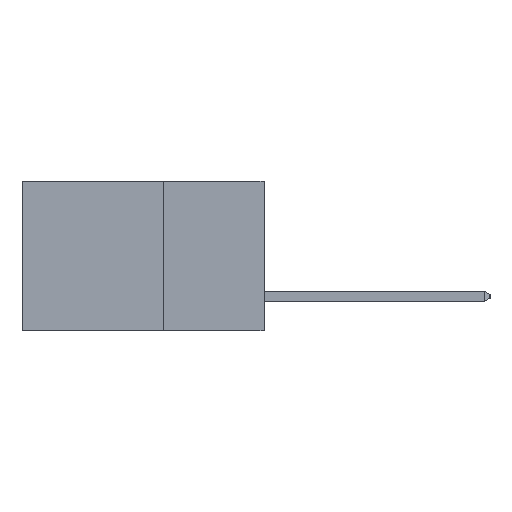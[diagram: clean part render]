
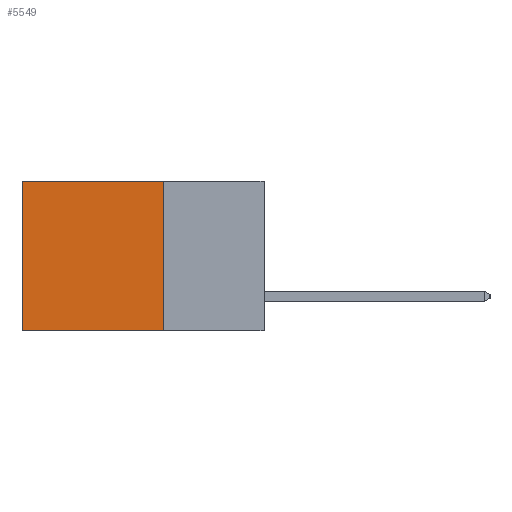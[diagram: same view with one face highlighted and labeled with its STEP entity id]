
A CAD part, left-side view. The second image highlights one B-rep face of the part: STEP entity #5549.
In plain terms, the highlighted planar face has unit normal (-1, 0, 0).
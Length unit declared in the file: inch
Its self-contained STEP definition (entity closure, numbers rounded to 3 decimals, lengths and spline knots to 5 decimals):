
#2765 = CARTESIAN_POINT ( 'NONE',  ( 0.298, 0.6, 0. ) ) ;
#3063 = CARTESIAN_POINT ( 'NONE',  ( 0.298, 0.25, -0.37 ) ) ;
#5543 = VERTEX_POINT ( 'NONE', #17831 ) ;
#5549 = ADVANCED_FACE ( 'NONE', ( #10870 ), #17980, .F. ) ;
#6004 = ORIENTED_EDGE ( 'NONE', *, *, #11829, .T. ) ;
#6258 = EDGE_LOOP ( 'NONE', ( #11097, #23341, #18489, #6004 ) ) ;
#6537 = VECTOR ( 'NONE', #27147, 39.37008 ) ;
#7311 = VECTOR ( 'NONE', #24824, 39.37008 ) ;
#10427 = CARTESIAN_POINT ( 'NONE',  ( 0.298, 0.25, 0. ) ) ;
#10778 = VERTEX_POINT ( 'NONE', #25812 ) ;
#10870 = FACE_OUTER_BOUND ( 'NONE', #6258, .T. ) ;
#11097 = ORIENTED_EDGE ( 'NONE', *, *, #23310, .T. ) ;
#11544 = LINE ( 'NONE', #10427, #22511 ) ;
#11580 = AXIS2_PLACEMENT_3D ( 'NONE', #17793, #17756, #17735 ) ;
#11829 = EDGE_CURVE ( 'NONE', #5543, #24438, #23789, .T. ) ;
#11945 = CARTESIAN_POINT ( 'NONE',  ( 0.298, 0.25, 0. ) ) ;
#12462 = LINE ( 'NONE', #2765, #23415 ) ;
#14728 = CARTESIAN_POINT ( 'NONE',  ( 0.298, 0.25, -0.37 ) ) ;
#15668 = EDGE_CURVE ( 'NONE', #22518, #10778, #18804, .T. ) ;
#16913 = CARTESIAN_POINT ( 'NONE',  ( 0.298, 0.6, 0. ) ) ;
#17231 = EDGE_CURVE ( 'NONE', #5543, #22518, #11544, .T. ) ;
#17735 = DIRECTION ( 'NONE',  ( 0., 0., -1. ) ) ;
#17756 = DIRECTION ( 'NONE',  ( 1., 0., 0. ) ) ;
#17793 = CARTESIAN_POINT ( 'NONE',  ( 0.298, 0.25, 0. ) ) ;
#17831 = CARTESIAN_POINT ( 'NONE',  ( 0.298, 0.25, 0. ) ) ;
#17858 = DIRECTION ( 'NONE',  ( 0., 0., -1. ) ) ;
#17980 = PLANE ( 'NONE',  #11580 ) ;
#18489 = ORIENTED_EDGE ( 'NONE', *, *, #17231, .F. ) ;
#18804 = LINE ( 'NONE', #3063, #7311 ) ;
#22511 = VECTOR ( 'NONE', #25669, 39.37008 ) ;
#22518 = VERTEX_POINT ( 'NONE', #14728 ) ;
#23310 = EDGE_CURVE ( 'NONE', #24438, #10778, #12462, .T. ) ;
#23341 = ORIENTED_EDGE ( 'NONE', *, *, #15668, .F. ) ;
#23415 = VECTOR ( 'NONE', #17858, 39.37008 ) ;
#23789 = LINE ( 'NONE', #11945, #6537 ) ;
#24438 = VERTEX_POINT ( 'NONE', #16913 ) ;
#24824 = DIRECTION ( 'NONE',  ( 0., 1., 0. ) ) ;
#25669 = DIRECTION ( 'NONE',  ( 0., 0., -1. ) ) ;
#25812 = CARTESIAN_POINT ( 'NONE',  ( 0.298, 0.6, -0.37 ) ) ;
#27147 = DIRECTION ( 'NONE',  ( 0., 1., 0. ) ) ;
